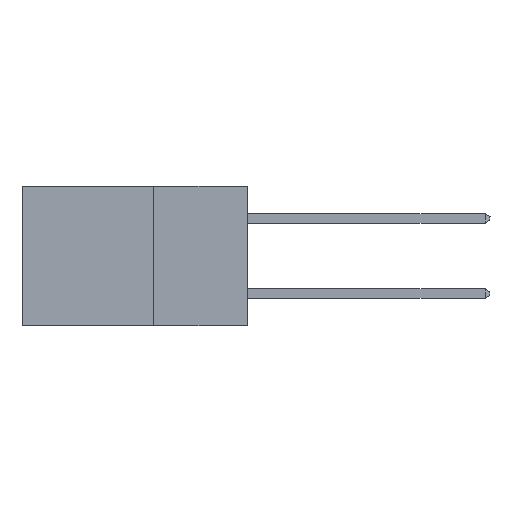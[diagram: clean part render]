
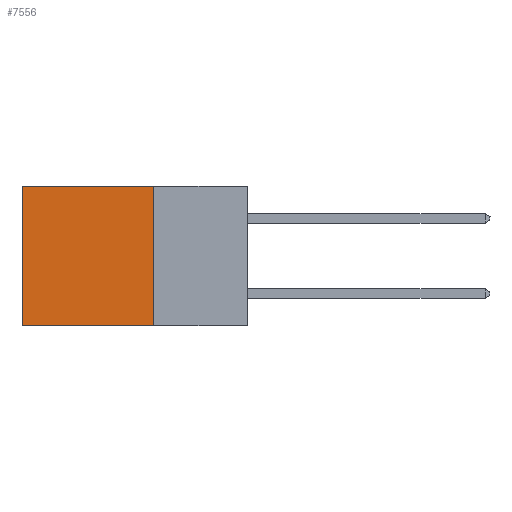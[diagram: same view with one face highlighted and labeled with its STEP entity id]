
A CAD part, left-side view. The second image highlights one B-rep face of the part: STEP entity #7556.
In plain terms, the highlighted planar face has unit normal (-1, 0, 0).
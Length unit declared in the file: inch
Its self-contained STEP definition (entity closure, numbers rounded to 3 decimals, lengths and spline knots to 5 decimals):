
#514 = ORIENTED_EDGE ( 'NONE', *, *, #15593, .F. ) ;
#1742 = LINE ( 'NONE', #13614, #12395 ) ;
#1769 = LINE ( 'NONE', #7557, #11329 ) ;
#2295 = VERTEX_POINT ( 'NONE', #7128 ) ;
#2333 = CARTESIAN_POINT ( 'NONE',  ( 0.2615, 0.25, 0. ) ) ;
#3133 = FACE_OUTER_BOUND ( 'NONE', #17320, .T. ) ;
#3661 = DIRECTION ( 'NONE',  ( 0., 1., 0. ) ) ;
#7128 = CARTESIAN_POINT ( 'NONE',  ( 0.2615, 0.25, -0.37 ) ) ;
#7415 = PLANE ( 'NONE',  #17655 ) ;
#7556 = ADVANCED_FACE ( 'NONE', ( #3133 ), #7415, .F. ) ;
#7557 = CARTESIAN_POINT ( 'NONE',  ( 0.2615, 0.6, -0.37 ) ) ;
#7831 = CARTESIAN_POINT ( 'NONE',  ( 0.2615, 0.25, -0.37 ) ) ;
#8400 = CARTESIAN_POINT ( 'NONE',  ( 0.2615, 0.25, 0. ) ) ;
#9028 = EDGE_CURVE ( 'NONE', #9326, #21732, #12336, .T. ) ;
#9326 = VERTEX_POINT ( 'NONE', #2333 ) ;
#9444 = DIRECTION ( 'NONE',  ( 0., 0., -1. ) ) ;
#9868 = CARTESIAN_POINT ( 'NONE',  ( 0.2615, 0.6, -0.37 ) ) ;
#11288 = EDGE_CURVE ( 'NONE', #21732, #16948, #1769, .T. ) ;
#11329 = VECTOR ( 'NONE', #17442, 39.37008 ) ;
#11791 = EDGE_CURVE ( 'NONE', #9326, #2295, #1742, .T. ) ;
#12336 = LINE ( 'NONE', #8400, #21313 ) ;
#12395 = VECTOR ( 'NONE', #9444, 39.37008 ) ;
#12766 = DIRECTION ( 'NONE',  ( 1., 0., 0. ) ) ;
#13614 = CARTESIAN_POINT ( 'NONE',  ( 0.2615, 0.25, -0.37 ) ) ;
#15294 = ORIENTED_EDGE ( 'NONE', *, *, #11288, .T. ) ;
#15593 = EDGE_CURVE ( 'NONE', #2295, #16948, #21013, .T. ) ;
#16681 = DIRECTION ( 'NONE',  ( 0., 0., -1. ) ) ;
#16948 = VERTEX_POINT ( 'NONE', #9868 ) ;
#17320 = EDGE_LOOP ( 'NONE', ( #15294, #514, #23049, #23492 ) ) ;
#17442 = DIRECTION ( 'NONE',  ( 0., 0., -1. ) ) ;
#17655 = AXIS2_PLACEMENT_3D ( 'NONE', #24410, #12766, #16681 ) ;
#18029 = CARTESIAN_POINT ( 'NONE',  ( 0.2615, 0.6, 0. ) ) ;
#20447 = DIRECTION ( 'NONE',  ( 0., 1., 0. ) ) ;
#21013 = LINE ( 'NONE', #7831, #24379 ) ;
#21313 = VECTOR ( 'NONE', #20447, 39.37008 ) ;
#21732 = VERTEX_POINT ( 'NONE', #18029 ) ;
#23049 = ORIENTED_EDGE ( 'NONE', *, *, #11791, .F. ) ;
#23492 = ORIENTED_EDGE ( 'NONE', *, *, #9028, .T. ) ;
#24379 = VECTOR ( 'NONE', #3661, 39.37008 ) ;
#24410 = CARTESIAN_POINT ( 'NONE',  ( 0.2615, 0.25, -0.37 ) ) ;
